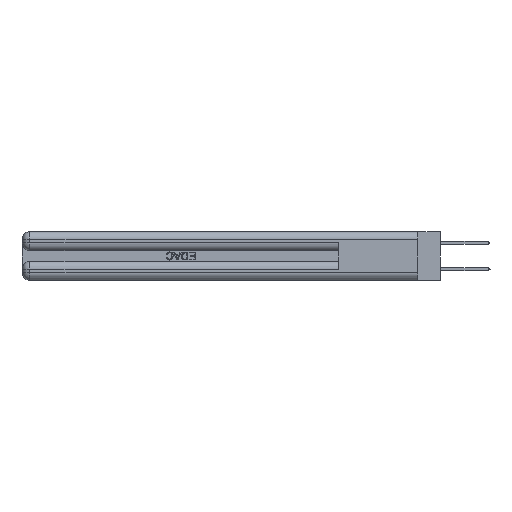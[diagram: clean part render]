
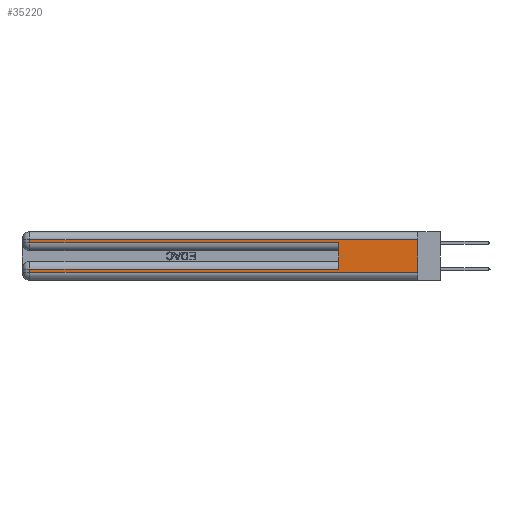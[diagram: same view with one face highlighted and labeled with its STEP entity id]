
A CAD part, left-side view. The second image highlights one B-rep face of the part: STEP entity #35220.
In plain terms, the highlighted planar face has unit normal (-1, 0, 0).
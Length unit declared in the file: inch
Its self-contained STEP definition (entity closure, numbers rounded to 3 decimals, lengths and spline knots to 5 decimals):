
#71 = VERTEX_POINT ( 'NONE', #8383 ) ;
#1059 = LINE ( 'NONE', #36829, #30636 ) ;
#1948 = ORIENTED_EDGE ( 'NONE', *, *, #37468, .F. ) ;
#2258 = CARTESIAN_POINT ( 'NONE',  ( 0., 0., 0.285 ) ) ;
#2481 = LINE ( 'NONE', #17706, #43907 ) ;
#4080 = DIRECTION ( 'NONE',  ( 0., -1., 0. ) ) ;
#4269 = CARTESIAN_POINT ( 'NONE',  ( 0., 0.6, 0.145 ) ) ;
#6633 = LINE ( 'NONE', #15835, #47999 ) ;
#7372 = CARTESIAN_POINT ( 'NONE',  ( 0., 0., 0.31 ) ) ;
#8383 = CARTESIAN_POINT ( 'NONE',  ( 0., 2.94, 0.085 ) ) ;
#8752 = DIRECTION ( 'NONE',  ( 0., 0., -1. ) ) ;
#8882 = CARTESIAN_POINT ( 'NONE',  ( 0., 2.94, 0.06 ) ) ;
#9933 = VERTEX_POINT ( 'NONE', #32663 ) ;
#10428 = VECTOR ( 'NONE', #28322, 39.37008 ) ;
#11174 = ORIENTED_EDGE ( 'NONE', *, *, #18897, .T. ) ;
#12540 = VECTOR ( 'NONE', #4080, 39.37008 ) ;
#12917 = CARTESIAN_POINT ( 'NONE',  ( 0., 0., 0.06 ) ) ;
#13180 = VERTEX_POINT ( 'NONE', #42436 ) ;
#13702 = DIRECTION ( 'NONE',  ( 0., 0., -1. ) ) ;
#13721 = CARTESIAN_POINT ( 'NONE',  ( 0., 2.94, 0.285 ) ) ;
#13814 = LINE ( 'NONE', #12917, #12540 ) ;
#14899 = DIRECTION ( 'NONE',  ( 1., 0., 0. ) ) ;
#15328 = CARTESIAN_POINT ( 'NONE',  ( 0., 2.94, 0.31 ) ) ;
#15835 = CARTESIAN_POINT ( 'NONE',  ( 0., 0., 0.085 ) ) ;
#15994 = FACE_OUTER_BOUND ( 'NONE', #17721, .T. ) ;
#16279 = VECTOR ( 'NONE', #30391, 39.37008 ) ;
#16832 = ORIENTED_EDGE ( 'NONE', *, *, #45958, .T. ) ;
#16936 = ORIENTED_EDGE ( 'NONE', *, *, #32326, .T. ) ;
#17295 = VERTEX_POINT ( 'NONE', #36533 ) ;
#17706 = CARTESIAN_POINT ( 'NONE',  ( 0., 2.94, 0.37 ) ) ;
#17721 = EDGE_LOOP ( 'NONE', ( #42569, #16936, #25088, #11174, #1948, #16832, #34083, #25459 ) ) ;
#18897 = EDGE_CURVE ( 'NONE', #42689, #17295, #36399, .T. ) ;
#19043 = VERTEX_POINT ( 'NONE', #46986 ) ;
#19873 = DIRECTION ( 'NONE',  ( 0., 1., 0. ) ) ;
#20613 = LINE ( 'NONE', #7372, #51276 ) ;
#25021 = CARTESIAN_POINT ( 'NONE',  ( 0., 2.94, 0.37 ) ) ;
#25088 = ORIENTED_EDGE ( 'NONE', *, *, #38910, .T. ) ;
#25459 = ORIENTED_EDGE ( 'NONE', *, *, #43851, .T. ) ;
#26360 = AXIS2_PLACEMENT_3D ( 'NONE', #50756, #14899, #42877 ) ;
#27799 = LINE ( 'NONE', #25021, #47843 ) ;
#28322 = DIRECTION ( 'NONE',  ( 0., 0., 1. ) ) ;
#28511 = VERTEX_POINT ( 'NONE', #8882 ) ;
#29044 = DIRECTION ( 'NONE',  ( 0., 0., -1. ) ) ;
#30391 = DIRECTION ( 'NONE',  ( 0., -1., 0. ) ) ;
#30636 = VECTOR ( 'NONE', #8752, 39.37008 ) ;
#32326 = EDGE_CURVE ( 'NONE', #9933, #39845, #20613, .T. ) ;
#32559 = EDGE_CURVE ( 'NONE', #9933, #13180, #1059, .T. ) ;
#32663 = CARTESIAN_POINT ( 'NONE',  ( 0., 0., 0.31 ) ) ;
#34083 = ORIENTED_EDGE ( 'NONE', *, *, #51074, .T. ) ;
#35220 = ADVANCED_FACE ( 'NONE', ( #15994 ), #38880, .F. ) ;
#36399 = LINE ( 'NONE', #2258, #16279 ) ;
#36533 = CARTESIAN_POINT ( 'NONE',  ( 0., 0.6, 0.285 ) ) ;
#36829 = CARTESIAN_POINT ( 'NONE',  ( 0., 0., 0.37 ) ) ;
#37468 = EDGE_CURVE ( 'NONE', #19043, #17295, #51768, .T. ) ;
#38880 = PLANE ( 'NONE',  #26360 ) ;
#38910 = EDGE_CURVE ( 'NONE', #39845, #42689, #27799, .T. ) ;
#39447 = DIRECTION ( 'NONE',  ( 0., 1., 0. ) ) ;
#39845 = VERTEX_POINT ( 'NONE', #15328 ) ;
#42436 = CARTESIAN_POINT ( 'NONE',  ( 0., 0., 0.06 ) ) ;
#42569 = ORIENTED_EDGE ( 'NONE', *, *, #32559, .F. ) ;
#42689 = VERTEX_POINT ( 'NONE', #13721 ) ;
#42877 = DIRECTION ( 'NONE',  ( 0., 0., -1. ) ) ;
#43851 = EDGE_CURVE ( 'NONE', #28511, #13180, #13814, .T. ) ;
#43907 = VECTOR ( 'NONE', #13702, 39.37008 ) ;
#45958 = EDGE_CURVE ( 'NONE', #19043, #71, #6633, .T. ) ;
#46986 = CARTESIAN_POINT ( 'NONE',  ( 0., 0.6, 0.085 ) ) ;
#47843 = VECTOR ( 'NONE', #29044, 39.37008 ) ;
#47999 = VECTOR ( 'NONE', #19873, 39.37008 ) ;
#50756 = CARTESIAN_POINT ( 'NONE',  ( 0., 0., 0.37 ) ) ;
#51074 = EDGE_CURVE ( 'NONE', #71, #28511, #2481, .T. ) ;
#51276 = VECTOR ( 'NONE', #39447, 39.37008 ) ;
#51768 = LINE ( 'NONE', #4269, #10428 ) ;
